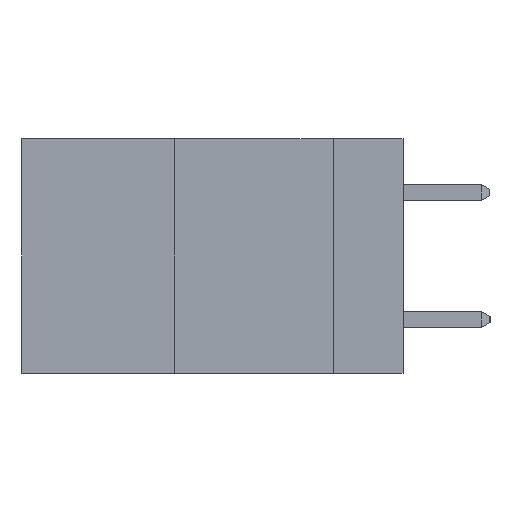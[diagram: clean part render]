
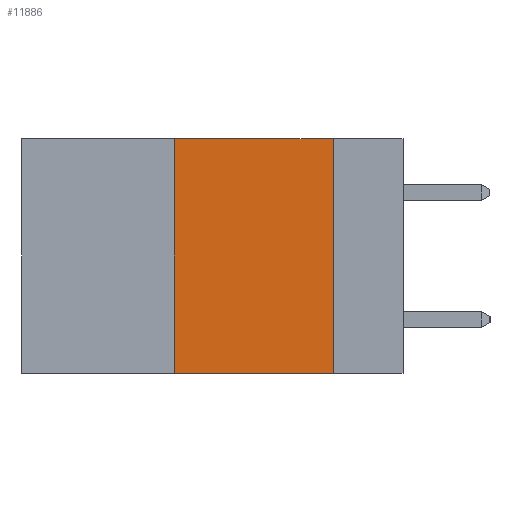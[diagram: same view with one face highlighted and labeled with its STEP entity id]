
A CAD part, left-side view. The second image highlights one B-rep face of the part: STEP entity #11886.
In plain terms, the highlighted planar face has unit normal (-1, 0, 0).
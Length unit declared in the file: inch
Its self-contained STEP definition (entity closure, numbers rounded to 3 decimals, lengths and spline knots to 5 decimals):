
#653 = VECTOR ( 'NONE', #6530, 39.37008 ) ;
#683 = DIRECTION ( 'NONE',  ( 0., -1., 0. ) ) ;
#692 = EDGE_CURVE ( 'NONE', #11177, #9833, #13006, .T. ) ;
#852 = VERTEX_POINT ( 'NONE', #12902 ) ;
#1024 = CARTESIAN_POINT ( 'NONE',  ( 0., 0.11, 0. ) ) ;
#1462 = CARTESIAN_POINT ( 'NONE',  ( 0., 0.6, 0. ) ) ;
#1545 = ORIENTED_EDGE ( 'NONE', *, *, #7364, .T. ) ;
#1773 = EDGE_CURVE ( 'NONE', #9833, #14638, #14238, .T. ) ;
#1932 = LINE ( 'NONE', #8807, #653 ) ;
#2360 = CARTESIAN_POINT ( 'NONE',  ( 0., 0.6, 0. ) ) ;
#2700 = CARTESIAN_POINT ( 'NONE',  ( 0., 0.11, 0. ) ) ;
#2783 = LINE ( 'NONE', #6324, #4540 ) ;
#2976 = VECTOR ( 'NONE', #6764, 39.37008 ) ;
#4540 = VECTOR ( 'NONE', #683, 39.37008 ) ;
#4833 = DIRECTION ( 'NONE',  ( 0., 0., -1. ) ) ;
#5674 = FACE_OUTER_BOUND ( 'NONE', #14540, .T. ) ;
#5847 = EDGE_CURVE ( 'NONE', #852, #11177, #1932, .T. ) ;
#5930 = ORIENTED_EDGE ( 'NONE', *, *, #1773, .F. ) ;
#6233 = CARTESIAN_POINT ( 'NONE',  ( 0., 0.11, -0.37 ) ) ;
#6324 = CARTESIAN_POINT ( 'NONE',  ( 0., 0.6, -0.37 ) ) ;
#6530 = DIRECTION ( 'NONE',  ( 0., 0., 1. ) ) ;
#6764 = DIRECTION ( 'NONE',  ( 0., -1., 0. ) ) ;
#7364 = EDGE_CURVE ( 'NONE', #852, #14638, #2783, .T. ) ;
#7384 = VECTOR ( 'NONE', #12381, 39.37008 ) ;
#8807 = CARTESIAN_POINT ( 'NONE',  ( 0., 0.36, 0. ) ) ;
#9381 = PLANE ( 'NONE',  #10704 ) ;
#9833 = VERTEX_POINT ( 'NONE', #2700 ) ;
#10073 = ORIENTED_EDGE ( 'NONE', *, *, #5847, .F. ) ;
#10704 = AXIS2_PLACEMENT_3D ( 'NONE', #1462, #11712, #4833 ) ;
#11177 = VERTEX_POINT ( 'NONE', #11546 ) ;
#11546 = CARTESIAN_POINT ( 'NONE',  ( 0., 0.36, 0. ) ) ;
#11712 = DIRECTION ( 'NONE',  ( 1., 0., 0. ) ) ;
#11886 = ADVANCED_FACE ( 'NONE', ( #5674 ), #9381, .F. ) ;
#12381 = DIRECTION ( 'NONE',  ( 0., 0., -1. ) ) ;
#12746 = ORIENTED_EDGE ( 'NONE', *, *, #692, .F. ) ;
#12902 = CARTESIAN_POINT ( 'NONE',  ( 0., 0.36, -0.37 ) ) ;
#13006 = LINE ( 'NONE', #2360, #2976 ) ;
#14238 = LINE ( 'NONE', #1024, #7384 ) ;
#14540 = EDGE_LOOP ( 'NONE', ( #5930, #12746, #10073, #1545 ) ) ;
#14638 = VERTEX_POINT ( 'NONE', #6233 ) ;
